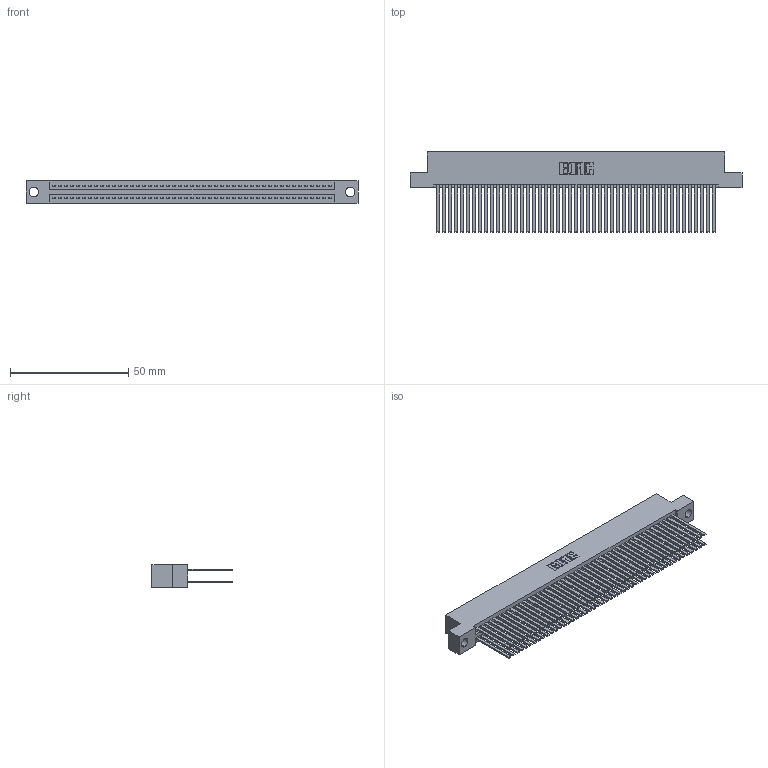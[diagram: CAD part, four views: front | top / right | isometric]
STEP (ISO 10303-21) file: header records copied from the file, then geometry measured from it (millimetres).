
FILE_DESCRIPTION (( 'STEP AP203' ), '1' );
FILE_NAME ('395-094-544-204.STEP', '2018-11-29T12:55:33', ( '' ), ( '' ), 'SwSTEP 2.0', 'SolidWorks 2016', '' );
FILE_SCHEMA (( 'CONFIG_CONTROL_DESIGN' ));
Length unit declared in the file: inch
Products named in the file (3): 345 Part_Flush Mounting Lugs - 0.156 Dia-TH; 345-292-001_345-293-144; 395-094-544-204
Assembly tree (95 placements, depth 2):
  395-094-544-204
    345 Part_Flush Mounting Lugs - 0.156 Dia-TH
    345-292-001_345-293-144  x94
Bounding box: 140.59 x 33.96 x 9.4 mm (x, y, z)
Volume: 14933.2 mm3; surface area: 25847.9 mm2
Topology: 95 solids, 95 shells, 4262 faces, 12655 edges, 8310 vertices
Faces by surface type: plane 2806, cylinder 1456
Entity records: 36023 total; most frequent: CARTESIAN_POINT 6032, ORIENTED_EDGE 5966, DIRECTION 5311, EDGE_CURVE 2983, LINE 2667, VECTOR 2667, VERTEX_POINT 1986, AXIS2_PLACEMENT_3D 1322
